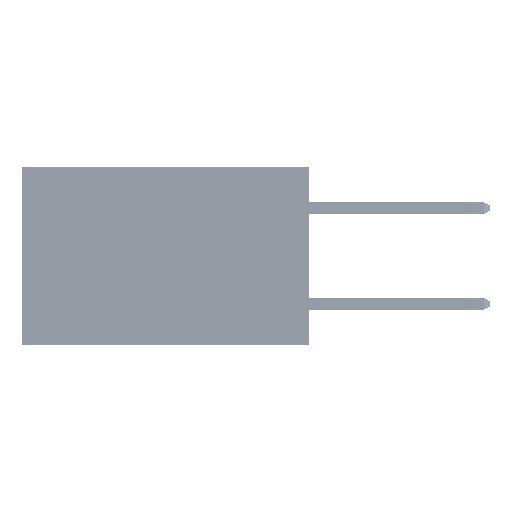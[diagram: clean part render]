
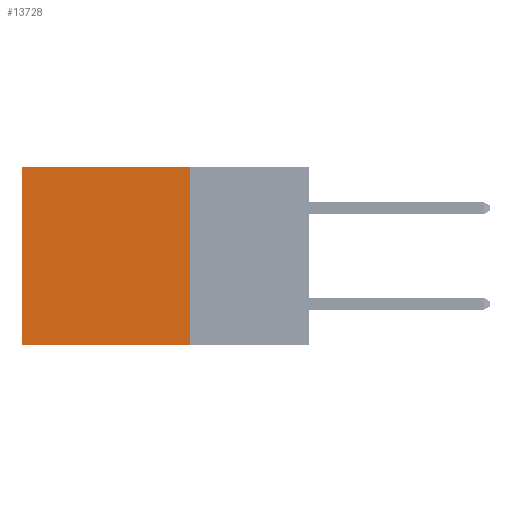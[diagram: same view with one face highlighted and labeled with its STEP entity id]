
A CAD part, left-side view. The second image highlights one B-rep face of the part: STEP entity #13728.
In plain terms, the highlighted planar face has unit normal (-1, 0, 0).
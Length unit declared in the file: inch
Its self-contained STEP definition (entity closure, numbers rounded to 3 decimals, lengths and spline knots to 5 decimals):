
#594 = VERTEX_POINT ( 'NONE', #27036 ) ;
#928 = CARTESIAN_POINT ( 'NONE',  ( 0.2875, 0.25, 0. ) ) ;
#1244 = DIRECTION ( 'NONE',  ( 0., 0., -1. ) ) ;
#1808 = CARTESIAN_POINT ( 'NONE',  ( 0.2875, 0.6, 0. ) ) ;
#2554 = EDGE_CURVE ( 'NONE', #594, #21881, #31080, .T. ) ;
#5460 = CARTESIAN_POINT ( 'NONE',  ( 0.2875, 0.25, 0. ) ) ;
#6810 = CARTESIAN_POINT ( 'NONE',  ( 0.2875, 0.25, -0.37 ) ) ;
#7284 = CARTESIAN_POINT ( 'NONE',  ( 0.2875, 0.6, 0. ) ) ;
#7379 = DIRECTION ( 'NONE',  ( 0., 1., 0. ) ) ;
#10274 = EDGE_LOOP ( 'NONE', ( #12732, #35707, #12081, #34983 ) ) ;
#12081 = ORIENTED_EDGE ( 'NONE', *, *, #21134, .F. ) ;
#12732 = ORIENTED_EDGE ( 'NONE', *, *, #33995, .T. ) ;
#13728 = ADVANCED_FACE ( 'NONE', ( #39360 ), #38388, .F. ) ;
#16409 = EDGE_CURVE ( 'NONE', #28850, #46885, #43212, .T. ) ;
#18541 = AXIS2_PLACEMENT_3D ( 'NONE', #45182, #23309, #1244 ) ;
#18879 = LINE ( 'NONE', #5460, #29326 ) ;
#21134 = EDGE_CURVE ( 'NONE', #28850, #594, #18879, .T. ) ;
#21236 = VECTOR ( 'NONE', #7379, 39.37008 ) ;
#21881 = VERTEX_POINT ( 'NONE', #24752 ) ;
#23053 = CARTESIAN_POINT ( 'NONE',  ( 0.2875, 0.25, 0. ) ) ;
#23309 = DIRECTION ( 'NONE',  ( 1., 0., 0. ) ) ;
#24752 = CARTESIAN_POINT ( 'NONE',  ( 0.2875, 0.6, -0.37 ) ) ;
#26255 = DIRECTION ( 'NONE',  ( 0., 1., 0. ) ) ;
#27036 = CARTESIAN_POINT ( 'NONE',  ( 0.2875, 0.25, -0.37 ) ) ;
#28850 = VERTEX_POINT ( 'NONE', #23053 ) ;
#29326 = VECTOR ( 'NONE', #31260, 39.37008 ) ;
#30874 = DIRECTION ( 'NONE',  ( 0., 0., -1. ) ) ;
#31080 = LINE ( 'NONE', #6810, #21236 ) ;
#31260 = DIRECTION ( 'NONE',  ( 0., 0., -1. ) ) ;
#33306 = VECTOR ( 'NONE', #26255, 39.37008 ) ;
#33995 = EDGE_CURVE ( 'NONE', #46885, #21881, #42366, .T. ) ;
#34983 = ORIENTED_EDGE ( 'NONE', *, *, #16409, .T. ) ;
#35707 = ORIENTED_EDGE ( 'NONE', *, *, #2554, .F. ) ;
#38388 = PLANE ( 'NONE',  #18541 ) ;
#39360 = FACE_OUTER_BOUND ( 'NONE', #10274, .T. ) ;
#42366 = LINE ( 'NONE', #1808, #44066 ) ;
#43212 = LINE ( 'NONE', #928, #33306 ) ;
#44066 = VECTOR ( 'NONE', #30874, 39.37008 ) ;
#45182 = CARTESIAN_POINT ( 'NONE',  ( 0.2875, 0.25, 0. ) ) ;
#46885 = VERTEX_POINT ( 'NONE', #7284 ) ;
